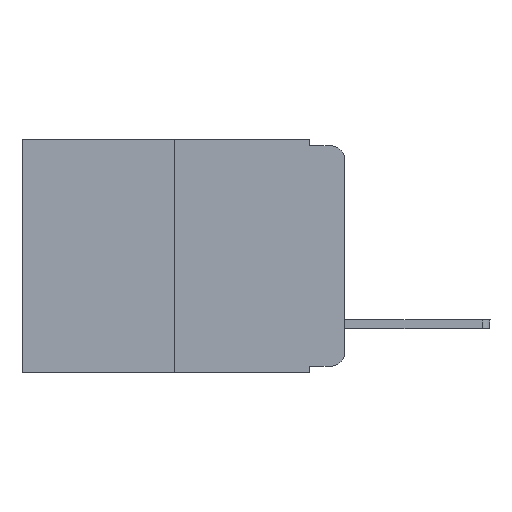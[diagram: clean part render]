
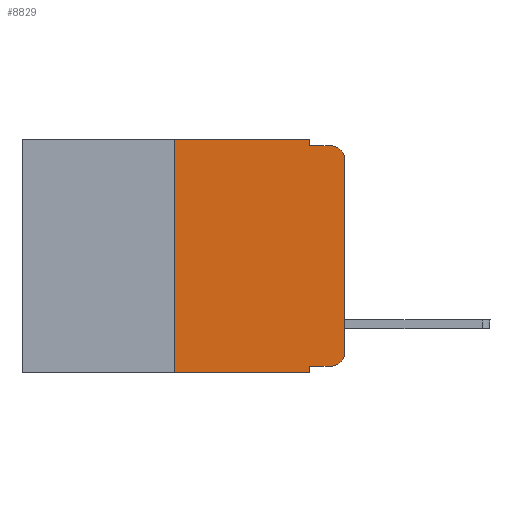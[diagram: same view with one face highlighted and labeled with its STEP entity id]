
A CAD part, left-side view. The second image highlights one B-rep face of the part: STEP entity #8829.
In plain terms, the highlighted planar face has unit normal (-1, 0, 0).
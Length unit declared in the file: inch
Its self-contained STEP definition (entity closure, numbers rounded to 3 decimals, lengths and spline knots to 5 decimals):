
#350 = VECTOR ( 'NONE', #2500, 39.37008 ) ;
#453 = LINE ( 'NONE', #10051, #350 ) ;
#487 = VERTEX_POINT ( 'NONE', #3230 ) ;
#629 = EDGE_CURVE ( 'NONE', #10517, #805, #4103, .T. ) ;
#805 = VERTEX_POINT ( 'NONE', #9753 ) ;
#938 = CARTESIAN_POINT ( 'NONE',  ( 0., 0., -0.313 ) ) ;
#1007 = LINE ( 'NONE', #1835, #10833 ) ;
#1068 = CIRCLE ( 'NONE', #11116, 0.02 ) ;
#1341 = CARTESIAN_POINT ( 'NONE',  ( 0., 0., 0. ) ) ;
#1460 = VERTEX_POINT ( 'NONE', #2371 ) ;
#1639 = ORIENTED_EDGE ( 'NONE', *, *, #12269, .F. ) ;
#1714 = CARTESIAN_POINT ( 'NONE',  ( 0., 0.051, -0.01 ) ) ;
#1835 = CARTESIAN_POINT ( 'NONE',  ( 0., 0.051, 0. ) ) ;
#2005 = DIRECTION ( 'NONE',  ( 0., 0., -1. ) ) ;
#2110 = CARTESIAN_POINT ( 'NONE',  ( 0., 0.051, -0.343 ) ) ;
#2118 = ORIENTED_EDGE ( 'NONE', *, *, #629, .T. ) ;
#2295 = AXIS2_PLACEMENT_3D ( 'NONE', #8289, #2708, #10123 ) ;
#2371 = CARTESIAN_POINT ( 'NONE',  ( 0., 0.25, 0. ) ) ;
#2500 = DIRECTION ( 'NONE',  ( 0., -1., 0. ) ) ;
#2577 = VERTEX_POINT ( 'NONE', #9646 ) ;
#2702 = ORIENTED_EDGE ( 'NONE', *, *, #9413, .T. ) ;
#2706 = EDGE_CURVE ( 'NONE', #10772, #10517, #5294, .T. ) ;
#2708 = DIRECTION ( 'NONE',  ( -1., 0., 0. ) ) ;
#2727 = DIRECTION ( 'NONE',  ( 0., -1., 0. ) ) ;
#2857 = ORIENTED_EDGE ( 'NONE', *, *, #8503, .T. ) ;
#2866 = VERTEX_POINT ( 'NONE', #1714 ) ;
#2944 = LINE ( 'NONE', #9735, #10634 ) ;
#3230 = CARTESIAN_POINT ( 'NONE',  ( 0., 0.25, -0.343 ) ) ;
#3421 = EDGE_CURVE ( 'NONE', #487, #1460, #11398, .T. ) ;
#3482 = ORIENTED_EDGE ( 'NONE', *, *, #4953, .T. ) ;
#3485 = ORIENTED_EDGE ( 'NONE', *, *, #7591, .F. ) ;
#3513 = DIRECTION ( 'NONE',  ( 0., 0., 1. ) ) ;
#3612 = ORIENTED_EDGE ( 'NONE', *, *, #5911, .F. ) ;
#3665 = LINE ( 'NONE', #7493, #4556 ) ;
#3714 = DIRECTION ( 'NONE',  ( 0., 0., -1. ) ) ;
#3821 = CARTESIAN_POINT ( 'NONE',  ( 0., 0.051, -0.333 ) ) ;
#3850 = FACE_OUTER_BOUND ( 'NONE', #6300, .T. ) ;
#3909 = CARTESIAN_POINT ( 'NONE',  ( 0., 0.473, 0. ) ) ;
#3989 = EDGE_CURVE ( 'NONE', #2866, #805, #4985, .T. ) ;
#4103 = CIRCLE ( 'NONE', #2295, 0.02 ) ;
#4556 = VECTOR ( 'NONE', #2727, 39.37008 ) ;
#4651 = PLANE ( 'NONE',  #10519 ) ;
#4731 = CARTESIAN_POINT ( 'NONE',  ( 0., 0.051, 0. ) ) ;
#4855 = DIRECTION ( 'NONE',  ( 0., -1., 0. ) ) ;
#4929 = VECTOR ( 'NONE', #5167, 39.37008 ) ;
#4953 = EDGE_CURVE ( 'NONE', #10479, #2577, #453, .T. ) ;
#4985 = LINE ( 'NONE', #8844, #5165 ) ;
#5165 = VECTOR ( 'NONE', #9839, 39.37008 ) ;
#5167 = DIRECTION ( 'NONE',  ( 0., 0., 1. ) ) ;
#5294 = LINE ( 'NONE', #1341, #4929 ) ;
#5587 = CARTESIAN_POINT ( 'NONE',  ( 0., 0.02, -0.313 ) ) ;
#5911 = EDGE_CURVE ( 'NONE', #12202, #2866, #1007, .T. ) ;
#6300 = EDGE_LOOP ( 'NONE', ( #12018, #2118, #11762, #3612, #1639, #12262, #2857, #3485, #3482, #2702 ) ) ;
#6732 = DIRECTION ( 'NONE',  ( 1., 0., 0. ) ) ;
#6749 = CARTESIAN_POINT ( 'NONE',  ( 0., 0.473, 0. ) ) ;
#6843 = DIRECTION ( 'NONE',  ( 0., 0., -1. ) ) ;
#6982 = VECTOR ( 'NONE', #4855, 39.37008 ) ;
#7493 = CARTESIAN_POINT ( 'NONE',  ( 0., 0.473, -0.343 ) ) ;
#7591 = EDGE_CURVE ( 'NONE', #10479, #10511, #2944, .T. ) ;
#7812 = LINE ( 'NONE', #6749, #6982 ) ;
#8280 = CARTESIAN_POINT ( 'NONE',  ( 0., 0.25, 0. ) ) ;
#8289 = CARTESIAN_POINT ( 'NONE',  ( 0., 0.02, -0.03 ) ) ;
#8503 = EDGE_CURVE ( 'NONE', #487, #10511, #3665, .T. ) ;
#8731 = DIRECTION ( 'NONE',  ( -1., 0., 0. ) ) ;
#8829 = ADVANCED_FACE ( 'NONE', ( #3850 ), #4651, .F. ) ;
#8844 = CARTESIAN_POINT ( 'NONE',  ( 0., 0.051, -0.01 ) ) ;
#9413 = EDGE_CURVE ( 'NONE', #2577, #10772, #1068, .T. ) ;
#9646 = CARTESIAN_POINT ( 'NONE',  ( 0., 0.02, -0.333 ) ) ;
#9735 = CARTESIAN_POINT ( 'NONE',  ( 0., 0.051, 0. ) ) ;
#9753 = CARTESIAN_POINT ( 'NONE',  ( 0., 0.02, -0.01 ) ) ;
#9839 = DIRECTION ( 'NONE',  ( 0., -1., 0. ) ) ;
#10051 = CARTESIAN_POINT ( 'NONE',  ( 0., 0.051, -0.333 ) ) ;
#10123 = DIRECTION ( 'NONE',  ( 0., 0., -1. ) ) ;
#10479 = VERTEX_POINT ( 'NONE', #3821 ) ;
#10511 = VERTEX_POINT ( 'NONE', #2110 ) ;
#10517 = VERTEX_POINT ( 'NONE', #11627 ) ;
#10519 = AXIS2_PLACEMENT_3D ( 'NONE', #3909, #6732, #3714 ) ;
#10634 = VECTOR ( 'NONE', #2005, 39.37008 ) ;
#10772 = VERTEX_POINT ( 'NONE', #938 ) ;
#10833 = VECTOR ( 'NONE', #11281, 39.37008 ) ;
#11116 = AXIS2_PLACEMENT_3D ( 'NONE', #5587, #8731, #6843 ) ;
#11281 = DIRECTION ( 'NONE',  ( 0., 0., -1. ) ) ;
#11398 = LINE ( 'NONE', #8280, #11407 ) ;
#11407 = VECTOR ( 'NONE', #3513, 39.37008 ) ;
#11627 = CARTESIAN_POINT ( 'NONE',  ( 0., 0., -0.03 ) ) ;
#11762 = ORIENTED_EDGE ( 'NONE', *, *, #3989, .F. ) ;
#12018 = ORIENTED_EDGE ( 'NONE', *, *, #2706, .T. ) ;
#12202 = VERTEX_POINT ( 'NONE', #4731 ) ;
#12262 = ORIENTED_EDGE ( 'NONE', *, *, #3421, .F. ) ;
#12269 = EDGE_CURVE ( 'NONE', #1460, #12202, #7812, .T. ) ;
